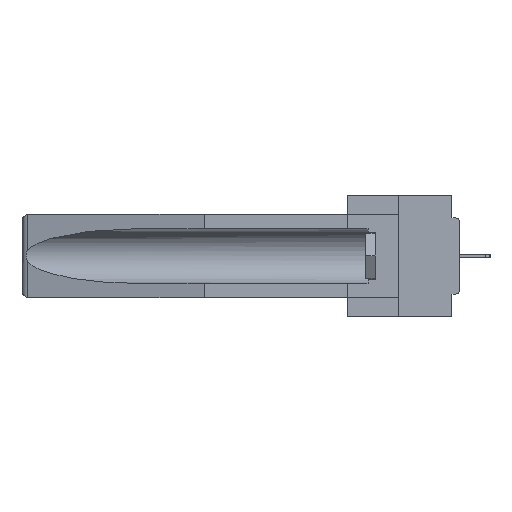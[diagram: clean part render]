
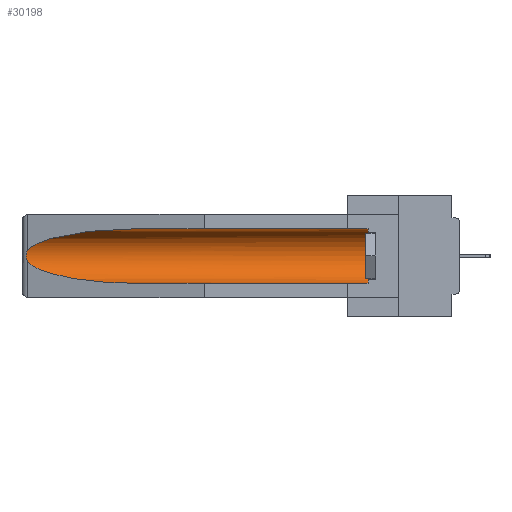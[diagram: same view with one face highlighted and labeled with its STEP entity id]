
A CAD part, left-side view. The second image highlights one B-rep face of the part: STEP entity #30198.
In plain terms, the highlighted cylindrical face has radius 2.857 mm (diameter 5.715 mm), a partial arc.
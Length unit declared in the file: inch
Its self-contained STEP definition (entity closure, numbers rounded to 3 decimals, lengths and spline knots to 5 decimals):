
#137 = CARTESIAN_POINT ( 'NONE',  ( 0.26537, 1.52718, -0.14972 ) ) ;
#788 = CARTESIAN_POINT ( 'NONE',  ( 0.26537, 1.52718, -0.14972 ) ) ;
#2011 = EDGE_CURVE ( 'NONE', #34672, #4661, #2720, .T. ) ;
#2042 = DIRECTION ( 'NONE',  ( 0., 0., 1. ) ) ;
#2338 = CARTESIAN_POINT ( 'NONE',  ( 0.155, 1.07973, -0.059 ) ) ;
#2720 = LINE ( 'NONE', #12427, #21818 ) ;
#3549 = CARTESIAN_POINT ( 'NONE',  ( 0.155, 0.126, -0.059 ) ) ;
#4210 = DIRECTION ( 'NONE',  ( 0., 1., 0. ) ) ;
#4661 = VERTEX_POINT ( 'NONE', #34128 ) ;
#5514 = DIRECTION ( 'NONE',  ( 0., 1., 0. ) ) ;
#6653 = CARTESIAN_POINT ( 'NONE',  ( 0.26655, 1.53094, -0.18657 ) ) ;
#7394 = CARTESIAN_POINT ( 'NONE',  ( 0.21114, 1.30732, -0.284 ) ) ;
#7532 = AXIS2_PLACEMENT_3D ( 'NONE', #27772, #18626, #30146 ) ;
#7822 = EDGE_CURVE ( 'NONE', #7973, #18379, #34247, .T. ) ;
#7973 = VERTEX_POINT ( 'NONE', #2338 ) ;
#9304 = ORIENTED_EDGE ( 'NONE', *, *, #2011, .F. ) ;
#9434 = CARTESIAN_POINT ( 'NONE',  ( 0.26537, 1.52718, -0.19328 ) ) ;
#9697 = CYLINDRICAL_SURFACE ( 'NONE', #7532, 0.1125 ) ;
#11063 = LINE ( 'NONE', #17209, #36696 ) ;
#12197 = CARTESIAN_POINT ( 'NONE',  ( 0.26597, 1.52961, -0.15275 ) ) ;
#12406 = CARTESIAN_POINT ( 'NONE',  ( 0.26597, 1.5296, -0.19026 ) ) ;
#12427 = CARTESIAN_POINT ( 'NONE',  ( 0.155, -0.30754, -0.284 ) ) ;
#12867 = FACE_OUTER_BOUND ( 'NONE', #38993, .T. ) ;
#12988 = ORIENTED_EDGE ( 'NONE', *, *, #31251, .T. ) ;
#14501 = CARTESIAN_POINT ( 'NONE',  ( 0.155, 1.07973, -0.284 ) ) ;
#14708 = DIRECTION ( 'NONE',  ( 0., -1., 0. ) ) ;
#14773 = AXIS2_PLACEMENT_3D ( 'NONE', #26429, #14708, #2042 ) ;
#17205 = EDGE_CURVE ( 'NONE', #38299, #4661, #35495, .T. ) ;
#17209 = CARTESIAN_POINT ( 'NONE',  ( 0.155, -0.30754, -0.059 ) ) ;
#18379 = VERTEX_POINT ( 'NONE', #27339 ) ;
#18626 = DIRECTION ( 'NONE',  ( 0., 1., 0. ) ) ;
#18780 = EDGE_CURVE ( 'NONE', #18379, #38299, #31929, .T. ) ;
#19643 = VERTEX_POINT ( 'NONE', #3549 ) ;
#21055 = CARTESIAN_POINT ( 'NONE',  ( 0.26537, 1.52718, -0.19328 ) ) ;
#21201 = CARTESIAN_POINT ( 'NONE',  ( 0.155, 0.126, -0.284 ) ) ;
#21818 = VECTOR ( 'NONE', #5514, 39.37008 ) ;
#22001 = EDGE_CURVE ( 'NONE', #34672, #19643, #37568, .T. ) ;
#22462 = CARTESIAN_POINT ( 'NONE',  ( 0.26537, 1.52718, -0.19328 ) ) ;
#24123 = CARTESIAN_POINT ( 'NONE',  ( 0.2673, 1.5327, -0.16383 ) ) ;
#24302 = CARTESIAN_POINT ( 'NONE',  ( 0.2675, 1.53308, -0.17534 ) ) ;
#26429 = CARTESIAN_POINT ( 'NONE',  ( 0.155, 0.126, -0.1715 ) ) ;
#27018 = ORIENTED_EDGE ( 'NONE', *, *, #18780, .T. ) ;
#27339 = CARTESIAN_POINT ( 'NONE',  ( 0.26537, 1.52718, -0.14972 ) ) ;
#27772 = CARTESIAN_POINT ( 'NONE',  ( 0.155, -0.30754, -0.1715 ) ) ;
#27946 = CARTESIAN_POINT ( 'NONE',  ( 0.155, 1.07973, -0.059 ) ) ;
#30146 = DIRECTION ( 'NONE',  ( 0., 0., 1. ) ) ;
#30198 = ADVANCED_FACE ( 'NONE', ( #12867 ), #9697, .F. ) ;
#30456 = CARTESIAN_POINT ( 'NONE',  ( 0.26654, 1.53092, -0.15636 ) ) ;
#30854 = CARTESIAN_POINT ( 'NONE',  ( 0.2675, 1.53308, -0.16763 ) ) ;
#31251 = EDGE_CURVE ( 'NONE', #19643, #7973, #11063, .T. ) ;
#31929 = B_SPLINE_CURVE_WITH_KNOTS ( 'NONE', 3,
 ( #137, #12197, #30456, #24123, #30854, #24302, #36197, #6653, #12406, #9434 ),
 .UNSPECIFIED., .F., .F.,
 ( 4, 2, 2, 2, 4 ),
 ( 0., 0.00029, 0.00058, 0.00087, 0.00117 ),
 .UNSPECIFIED. ) ;
#32312 = ORIENTED_EDGE ( 'NONE', *, *, #22001, .T. ) ;
#34128 = CARTESIAN_POINT ( 'NONE',  ( 0.155, 1.07973, -0.284 ) ) ;
#34247 =( BOUNDED_CURVE ( )  B_SPLINE_CURVE ( 3, ( #27946, #37042, #37834, #788 ),
 .UNSPECIFIED., .F., .F. ) 
 B_SPLINE_CURVE_WITH_KNOTS ( ( 4, 4 ),
 ( 4.71239, 6.08839 ),
 .UNSPECIFIED. ) 
 CURVE ( )  GEOMETRIC_REPRESENTATION_ITEM ( )  RATIONAL_B_SPLINE_CURVE ( ( 1., 0.848, 0.848, 1. ) ) 
 REPRESENTATION_ITEM ( '' )  );
#34563 = CARTESIAN_POINT ( 'NONE',  ( 0.25451, 1.48313, -0.24835 ) ) ;
#34672 = VERTEX_POINT ( 'NONE', #21201 ) ;
#35495 =( BOUNDED_CURVE ( )  B_SPLINE_CURVE ( 3, ( #22462, #34563, #7394, #14501 ),
 .UNSPECIFIED., .F., .F. ) 
 B_SPLINE_CURVE_WITH_KNOTS ( ( 4, 4 ),
 ( 0.1948, 1.5708 ),
 .UNSPECIFIED. ) 
 CURVE ( )  GEOMETRIC_REPRESENTATION_ITEM ( )  RATIONAL_B_SPLINE_CURVE ( ( 1., 0.848, 0.848, 1. ) ) 
 REPRESENTATION_ITEM ( '' )  );
#36197 = CARTESIAN_POINT ( 'NONE',  ( 0.2673, 1.53269, -0.17917 ) ) ;
#36696 = VECTOR ( 'NONE', #4210, 39.37008 ) ;
#37042 = CARTESIAN_POINT ( 'NONE',  ( 0.21114, 1.30732, -0.059 ) ) ;
#37568 = CIRCLE ( 'NONE', #14773, 0.1125 ) ;
#37834 = CARTESIAN_POINT ( 'NONE',  ( 0.25451, 1.48313, -0.09465 ) ) ;
#37905 = ORIENTED_EDGE ( 'NONE', *, *, #17205, .T. ) ;
#38299 = VERTEX_POINT ( 'NONE', #21055 ) ;
#38619 = ORIENTED_EDGE ( 'NONE', *, *, #7822, .T. ) ;
#38993 = EDGE_LOOP ( 'NONE', ( #38619, #27018, #37905, #9304, #32312, #12988 ) ) ;
